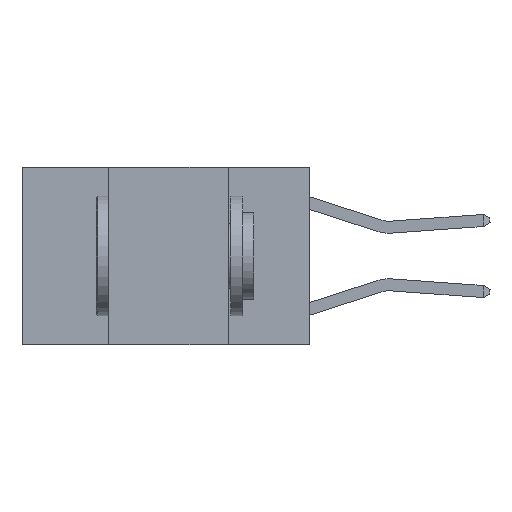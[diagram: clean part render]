
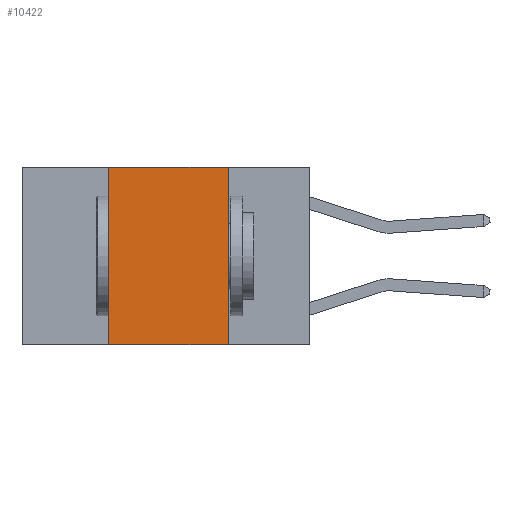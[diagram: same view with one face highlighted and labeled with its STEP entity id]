
A CAD part, left-side view. The second image highlights one B-rep face of the part: STEP entity #10422.
In plain terms, the highlighted planar face has unit normal (-1, 0, 0).
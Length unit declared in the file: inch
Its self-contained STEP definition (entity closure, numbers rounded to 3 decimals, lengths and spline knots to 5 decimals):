
#145 = CARTESIAN_POINT ( 'NONE',  ( 0., 0.17, 0. ) ) ;
#341 = DIRECTION ( 'NONE',  ( 0., 0., 1. ) ) ;
#356 = CARTESIAN_POINT ( 'NONE',  ( 0., 0.42, -0.37 ) ) ;
#980 = VECTOR ( 'NONE', #1264, 39.37008 ) ;
#1146 = VECTOR ( 'NONE', #7909, 39.37008 ) ;
#1254 = LINE ( 'NONE', #4510, #9845 ) ;
#1264 = DIRECTION ( 'NONE',  ( 0., -1., 0. ) ) ;
#1387 = CARTESIAN_POINT ( 'NONE',  ( 0., 0.6, -0.37 ) ) ;
#1399 = ORIENTED_EDGE ( 'NONE', *, *, #1832, .F. ) ;
#1475 = VERTEX_POINT ( 'NONE', #145 ) ;
#1611 = VERTEX_POINT ( 'NONE', #356 ) ;
#1676 = EDGE_CURVE ( 'NONE', #1611, #7245, #6398, .T. ) ;
#1832 = EDGE_CURVE ( 'NONE', #8788, #1475, #3738, .T. ) ;
#2631 = LINE ( 'NONE', #5866, #10200 ) ;
#3738 = LINE ( 'NONE', #8496, #980 ) ;
#4157 = DIRECTION ( 'NONE',  ( 0., 0., -1. ) ) ;
#4245 = AXIS2_PLACEMENT_3D ( 'NONE', #9491, #4629, #7899 ) ;
#4459 = CARTESIAN_POINT ( 'NONE',  ( 0., 0.17, -0.37 ) ) ;
#4510 = CARTESIAN_POINT ( 'NONE',  ( 0., 0.17, 0. ) ) ;
#4629 = DIRECTION ( 'NONE',  ( 1., 0., 0. ) ) ;
#4671 = ORIENTED_EDGE ( 'NONE', *, *, #8401, .F. ) ;
#5866 = CARTESIAN_POINT ( 'NONE',  ( 0., 0.42, 0. ) ) ;
#6228 = PLANE ( 'NONE',  #4245 ) ;
#6398 = LINE ( 'NONE', #1387, #1146 ) ;
#6495 = ORIENTED_EDGE ( 'NONE', *, *, #8424, .F. ) ;
#7245 = VERTEX_POINT ( 'NONE', #4459 ) ;
#7660 = CARTESIAN_POINT ( 'NONE',  ( 0., 0.42, 0. ) ) ;
#7899 = DIRECTION ( 'NONE',  ( 0., 0., -1. ) ) ;
#7909 = DIRECTION ( 'NONE',  ( 0., -1., 0. ) ) ;
#8141 = ORIENTED_EDGE ( 'NONE', *, *, #1676, .T. ) ;
#8401 = EDGE_CURVE ( 'NONE', #1611, #8788, #2631, .T. ) ;
#8424 = EDGE_CURVE ( 'NONE', #1475, #7245, #1254, .T. ) ;
#8496 = CARTESIAN_POINT ( 'NONE',  ( 0., 0.6, 0. ) ) ;
#8788 = VERTEX_POINT ( 'NONE', #7660 ) ;
#9491 = CARTESIAN_POINT ( 'NONE',  ( 0., 0.6, 0. ) ) ;
#9845 = VECTOR ( 'NONE', #4157, 39.37008 ) ;
#10200 = VECTOR ( 'NONE', #341, 39.37008 ) ;
#10277 = EDGE_LOOP ( 'NONE', ( #6495, #1399, #4671, #8141 ) ) ;
#10302 = FACE_OUTER_BOUND ( 'NONE', #10277, .T. ) ;
#10422 = ADVANCED_FACE ( 'NONE', ( #10302 ), #6228, .F. ) ;
